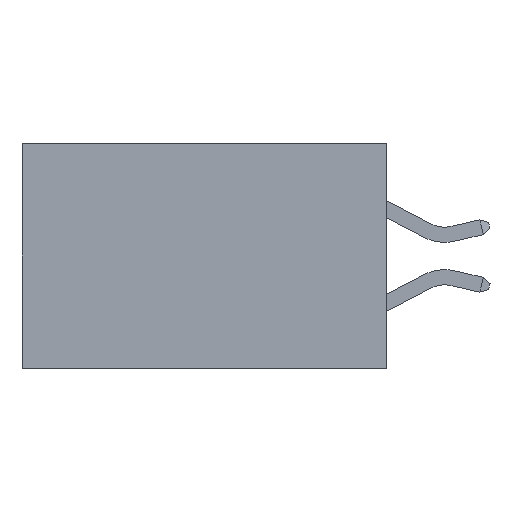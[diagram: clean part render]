
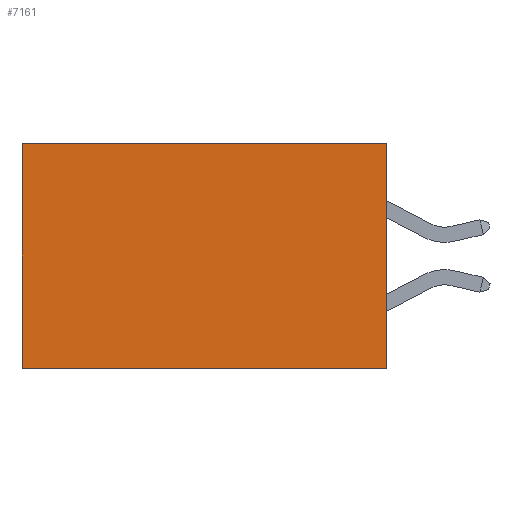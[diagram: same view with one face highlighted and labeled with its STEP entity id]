
A CAD part, left-side view. The second image highlights one B-rep face of the part: STEP entity #7161.
In plain terms, the highlighted planar face has unit normal (-1, 0, 0).
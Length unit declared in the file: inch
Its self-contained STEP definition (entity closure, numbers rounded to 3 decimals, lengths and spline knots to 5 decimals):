
#393 = EDGE_LOOP ( 'NONE', ( #3149, #5289, #8659, #9388 ) ) ;
#591 = PLANE ( 'NONE',  #9795 ) ;
#908 = DIRECTION ( 'NONE',  ( 0., 0., -1. ) ) ;
#1034 = EDGE_CURVE ( 'NONE', #3150, #8600, #1260, .T. ) ;
#1113 = LINE ( 'NONE', #2478, #6942 ) ;
#1260 = LINE ( 'NONE', #8449, #1601 ) ;
#1601 = VECTOR ( 'NONE', #3232, 39.37008 ) ;
#1803 = CARTESIAN_POINT ( 'NONE',  ( 0.298, 0., 0. ) ) ;
#1885 = CARTESIAN_POINT ( 'NONE',  ( 0.298, 0., -0.37 ) ) ;
#2086 = EDGE_CURVE ( 'NONE', #8149, #3150, #1113, .T. ) ;
#2478 = CARTESIAN_POINT ( 'NONE',  ( 0.298, 0., 0. ) ) ;
#2842 = CARTESIAN_POINT ( 'NONE',  ( 0.298, 0., 0. ) ) ;
#3090 = LINE ( 'NONE', #4055, #6674 ) ;
#3149 = ORIENTED_EDGE ( 'NONE', *, *, #9733, .T. ) ;
#3150 = VERTEX_POINT ( 'NONE', #1885 ) ;
#3232 = DIRECTION ( 'NONE',  ( 0., 1., 0. ) ) ;
#3538 = EDGE_CURVE ( 'NONE', #8149, #7356, #7917, .T. ) ;
#3595 = CARTESIAN_POINT ( 'NONE',  ( 0.298, 0.6, -0.37 ) ) ;
#4055 = CARTESIAN_POINT ( 'NONE',  ( 0.298, 0.6, 0. ) ) ;
#4951 = DIRECTION ( 'NONE',  ( 0., 1., 0. ) ) ;
#5103 = DIRECTION ( 'NONE',  ( 0., 0., -1. ) ) ;
#5289 = ORIENTED_EDGE ( 'NONE', *, *, #1034, .F. ) ;
#5545 = DIRECTION ( 'NONE',  ( 0., 0., -1. ) ) ;
#6674 = VECTOR ( 'NONE', #5545, 39.37008 ) ;
#6942 = VECTOR ( 'NONE', #908, 39.37008 ) ;
#7161 = ADVANCED_FACE ( 'NONE', ( #7479 ), #591, .F. ) ;
#7320 = VECTOR ( 'NONE', #4951, 39.37008 ) ;
#7356 = VERTEX_POINT ( 'NONE', #8579 ) ;
#7479 = FACE_OUTER_BOUND ( 'NONE', #393, .T. ) ;
#7917 = LINE ( 'NONE', #1803, #7320 ) ;
#8149 = VERTEX_POINT ( 'NONE', #8594 ) ;
#8449 = CARTESIAN_POINT ( 'NONE',  ( 0.298, 0., -0.37 ) ) ;
#8579 = CARTESIAN_POINT ( 'NONE',  ( 0.298, 0.6, 0. ) ) ;
#8594 = CARTESIAN_POINT ( 'NONE',  ( 0.298, 0., 0. ) ) ;
#8600 = VERTEX_POINT ( 'NONE', #3595 ) ;
#8659 = ORIENTED_EDGE ( 'NONE', *, *, #2086, .F. ) ;
#9388 = ORIENTED_EDGE ( 'NONE', *, *, #3538, .T. ) ;
#9705 = DIRECTION ( 'NONE',  ( 1., 0., 0. ) ) ;
#9733 = EDGE_CURVE ( 'NONE', #7356, #8600, #3090, .T. ) ;
#9795 = AXIS2_PLACEMENT_3D ( 'NONE', #2842, #9705, #5103 ) ;
